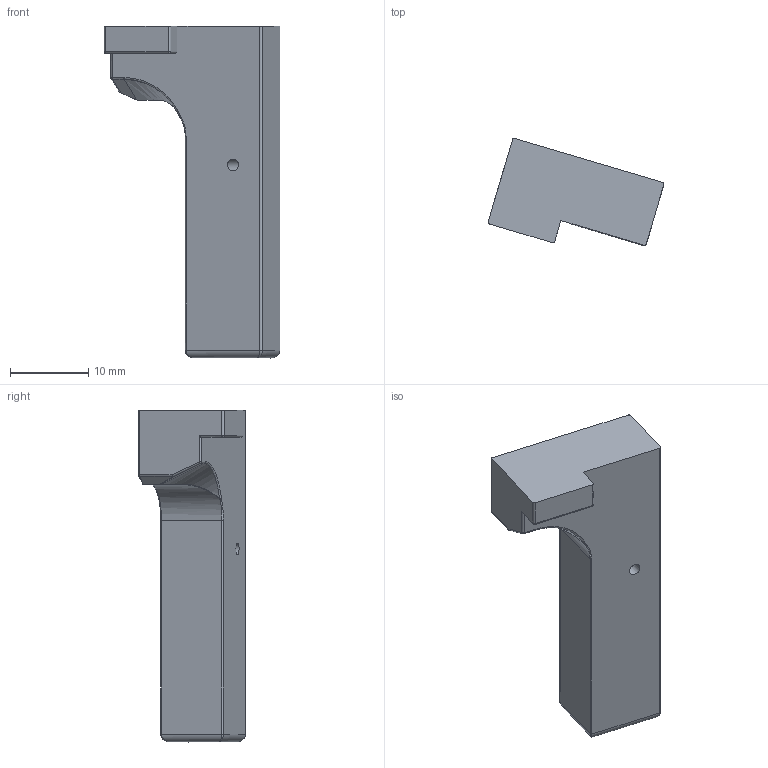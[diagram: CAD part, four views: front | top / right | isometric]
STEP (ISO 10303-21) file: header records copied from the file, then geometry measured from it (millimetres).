
FILE_DESCRIPTION (( 'STEP AP203' ), '1' );
FILE_NAME ('MOD9_mag_catch.STEP', '2020-06-10T04:59:46', ( '' ), ( '' ), 'SwSTEP 2.0', 'SolidWorks 2016', '' );
FILE_SCHEMA (( 'CONFIG_CONTROL_DESIGN' ));
Length unit declared in the file: millimetre
Products named in the file (1): MOD9_mag_catch
Bounding box: 22.43 x 13.63 x 42.38 mm (x, y, z)
Volume: 4466.2 mm3; surface area: 2144.5 mm2
Topology: 1 solids, 1 shells, 58 faces, 134 edges, 71 vertices
Faces by surface type: cylinder 24, bspline 14, plane 13, sphere 4, torus 3
Full cylindrical faces by diameter (mm): 1.5 x1
Entity records: 2066 total; most frequent: CARTESIAN_POINT 831, ORIENTED_EDGE 252, DIRECTION 211, EDGE_CURVE 126, AXIS2_PLACEMENT_3D 78, VERTEX_POINT 71, EDGE_LOOP 61, FACE_OUTER_BOUND 59
